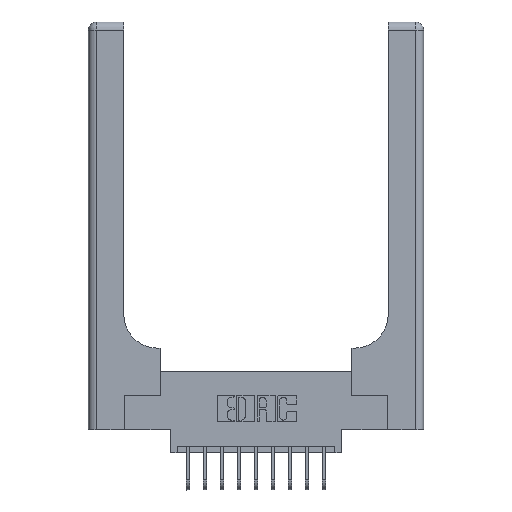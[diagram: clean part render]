
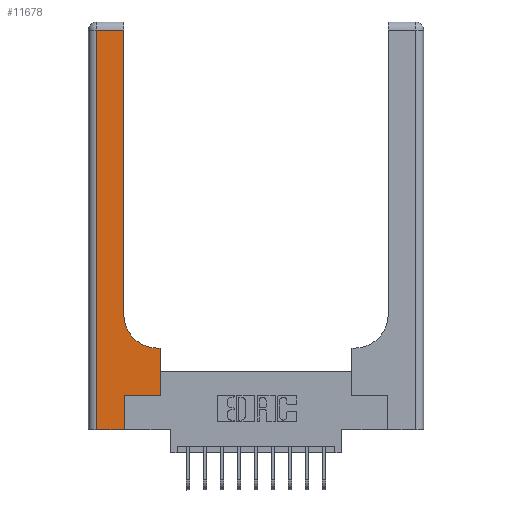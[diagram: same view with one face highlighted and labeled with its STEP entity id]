
A CAD part, top view. The second image highlights one B-rep face of the part: STEP entity #11678.
In plain terms, the highlighted planar face has unit normal (0, 0, 1).
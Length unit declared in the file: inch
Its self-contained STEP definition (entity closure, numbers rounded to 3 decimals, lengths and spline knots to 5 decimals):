
#762 = EDGE_CURVE ( 'NONE', #15086, #12486, #13425, .T. ) ;
#792 = VECTOR ( 'NONE', #10471, 39.37008 ) ;
#918 = DIRECTION ( 'NONE',  ( 0., 0., -1. ) ) ;
#1231 = VECTOR ( 'NONE', #6956, 39.37008 ) ;
#1309 = VECTOR ( 'NONE', #3744, 39.37008 ) ;
#1444 = LINE ( 'NONE', #13648, #8273 ) ;
#1561 = EDGE_CURVE ( 'NONE', #5451, #14541, #13488, .T. ) ;
#1607 = ORIENTED_EDGE ( 'NONE', *, *, #13177, .T. ) ;
#1825 = CARTESIAN_POINT ( 'NONE',  ( 0.51, 0.85, 0.37 ) ) ;
#2311 = CARTESIAN_POINT ( 'NONE',  ( 0.06, 0., 0.37 ) ) ;
#2360 = DIRECTION ( 'NONE',  ( -1., 0., 0. ) ) ;
#2430 = CARTESIAN_POINT ( 'NONE',  ( 0.528, 0.25, 0.37 ) ) ;
#2692 = EDGE_CURVE ( 'NONE', #14541, #10205, #14390, .T. ) ;
#2796 = DIRECTION ( 'NONE',  ( 0., 0., -1. ) ) ;
#3168 = CARTESIAN_POINT ( 'NONE',  ( 0.265, 0., 0.37 ) ) ;
#3477 = PLANE ( 'NONE',  #6799 ) ;
#3659 = CARTESIAN_POINT ( 'NONE',  ( 0.528, 0.6, 0.37 ) ) ;
#3744 = DIRECTION ( 'NONE',  ( 0., 1., 0. ) ) ;
#3911 = LINE ( 'NONE', #8799, #1309 ) ;
#4137 = VECTOR ( 'NONE', #5029, 39.37008 ) ;
#4315 = CARTESIAN_POINT ( 'NONE',  ( 0.26, 0.6, 0.37 ) ) ;
#4612 = CARTESIAN_POINT ( 'NONE',  ( 0., 3., 0.37 ) ) ;
#4792 = VERTEX_POINT ( 'NONE', #2311 ) ;
#5012 = EDGE_LOOP ( 'NONE', ( #12243, #14098, #11143, #1607, #12737, #15782, #15532, #9594, #6823 ) ) ;
#5029 = DIRECTION ( 'NONE',  ( 1., 0., 0. ) ) ;
#5107 = EDGE_CURVE ( 'NONE', #15145, #11149, #3911, .T. ) ;
#5130 = EDGE_CURVE ( 'NONE', #11149, #15086, #7907, .T. ) ;
#5148 = DIRECTION ( 'NONE',  ( -1., 0., 0. ) ) ;
#5215 = DIRECTION ( 'NONE',  ( 0., -1., 0. ) ) ;
#5224 = CARTESIAN_POINT ( 'NONE',  ( 0.26, 3., 0.37 ) ) ;
#5451 = VERTEX_POINT ( 'NONE', #7328 ) ;
#6329 = CARTESIAN_POINT ( 'NONE',  ( 0., 0., 0.37 ) ) ;
#6799 = AXIS2_PLACEMENT_3D ( 'NONE', #4612, #918, #2360 ) ;
#6823 = ORIENTED_EDGE ( 'NONE', *, *, #13391, .T. ) ;
#6956 = DIRECTION ( 'NONE',  ( -1., 0., 0. ) ) ;
#7328 = CARTESIAN_POINT ( 'NONE',  ( 0.26, 0.85, 0.37 ) ) ;
#7907 = LINE ( 'NONE', #10394, #792 ) ;
#7946 = VECTOR ( 'NONE', #5148, 39.37008 ) ;
#8182 = LINE ( 'NONE', #6329, #4137 ) ;
#8273 = VECTOR ( 'NONE', #5215, 39.37008 ) ;
#8601 = DIRECTION ( 'NONE',  ( 0., 1., 0. ) ) ;
#8617 = AXIS2_PLACEMENT_3D ( 'NONE', #1825, #2796, #10094 ) ;
#8799 = CARTESIAN_POINT ( 'NONE',  ( 0.265, 0., 0.37 ) ) ;
#9168 = CARTESIAN_POINT ( 'NONE',  ( 0.06, 2.94, 0.37 ) ) ;
#9321 = EDGE_CURVE ( 'NONE', #10205, #4792, #1444, .T. ) ;
#9594 = ORIENTED_EDGE ( 'NONE', *, *, #13461, .T. ) ;
#10094 = DIRECTION ( 'NONE',  ( 1., 0., 0. ) ) ;
#10181 = VERTEX_POINT ( 'NONE', #11568 ) ;
#10205 = VERTEX_POINT ( 'NONE', #9168 ) ;
#10394 = CARTESIAN_POINT ( 'NONE',  ( 0.265, 0.25, 0.37 ) ) ;
#10471 = DIRECTION ( 'NONE',  ( 1., 0., 0. ) ) ;
#10927 = FACE_OUTER_BOUND ( 'NONE', #5012, .T. ) ;
#11004 = DIRECTION ( 'NONE',  ( 0., 1., 0. ) ) ;
#11143 = ORIENTED_EDGE ( 'NONE', *, *, #9321, .T. ) ;
#11149 = VERTEX_POINT ( 'NONE', #14260 ) ;
#11568 = CARTESIAN_POINT ( 'NONE',  ( 0.51, 0.6, 0.37 ) ) ;
#11678 = ADVANCED_FACE ( 'NONE', ( #10927 ), #3477, .F. ) ;
#12243 = ORIENTED_EDGE ( 'NONE', *, *, #1561, .T. ) ;
#12486 = VERTEX_POINT ( 'NONE', #3659 ) ;
#12737 = ORIENTED_EDGE ( 'NONE', *, *, #5107, .T. ) ;
#12965 = CARTESIAN_POINT ( 'NONE',  ( 0.528, 0.25, 0.37 ) ) ;
#13056 = VECTOR ( 'NONE', #8601, 39.37008 ) ;
#13177 = EDGE_CURVE ( 'NONE', #4792, #15145, #8182, .T. ) ;
#13183 = CARTESIAN_POINT ( 'NONE',  ( 0., 2.94, 0.37 ) ) ;
#13391 = EDGE_CURVE ( 'NONE', #10181, #5451, #14258, .T. ) ;
#13425 = LINE ( 'NONE', #2430, #15088 ) ;
#13461 = EDGE_CURVE ( 'NONE', #12486, #10181, #15531, .T. ) ;
#13488 = LINE ( 'NONE', #5224, #13056 ) ;
#13648 = CARTESIAN_POINT ( 'NONE',  ( 0.06, 3., 0.37 ) ) ;
#13795 = CARTESIAN_POINT ( 'NONE',  ( 0.26, 2.94, 0.37 ) ) ;
#14098 = ORIENTED_EDGE ( 'NONE', *, *, #2692, .T. ) ;
#14258 = CIRCLE ( 'NONE', #8617, 0.25 ) ;
#14260 = CARTESIAN_POINT ( 'NONE',  ( 0.265, 0.25, 0.37 ) ) ;
#14390 = LINE ( 'NONE', #13183, #7946 ) ;
#14541 = VERTEX_POINT ( 'NONE', #13795 ) ;
#15086 = VERTEX_POINT ( 'NONE', #12965 ) ;
#15088 = VECTOR ( 'NONE', #11004, 39.37008 ) ;
#15145 = VERTEX_POINT ( 'NONE', #3168 ) ;
#15531 = LINE ( 'NONE', #4315, #1231 ) ;
#15532 = ORIENTED_EDGE ( 'NONE', *, *, #762, .T. ) ;
#15782 = ORIENTED_EDGE ( 'NONE', *, *, #5130, .T. ) ;
